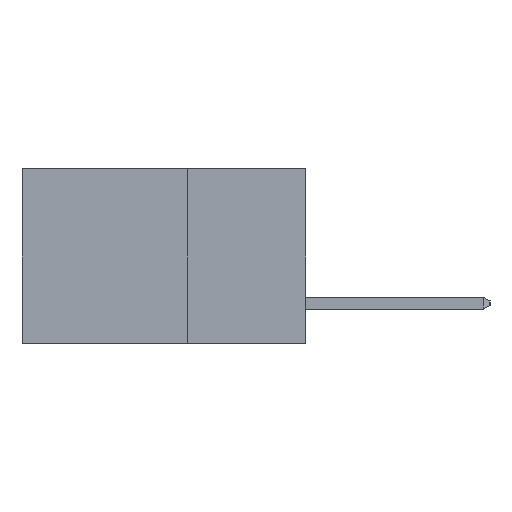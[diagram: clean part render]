
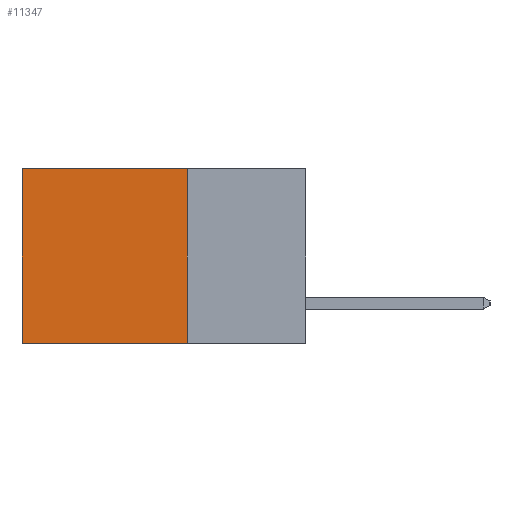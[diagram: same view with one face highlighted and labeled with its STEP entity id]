
A CAD part, left-side view. The second image highlights one B-rep face of the part: STEP entity #11347.
In plain terms, the highlighted planar face has unit normal (-1, 0, 0).
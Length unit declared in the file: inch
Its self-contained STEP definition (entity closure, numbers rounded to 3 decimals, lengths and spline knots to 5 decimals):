
#535 = EDGE_LOOP ( 'NONE', ( #16346, #4871, #7516, #13680 ) ) ;
#562 = CARTESIAN_POINT ( 'NONE',  ( 0.2615, 0.25, 0. ) ) ;
#1863 = EDGE_CURVE ( 'NONE', #21074, #2598, #10101, .T. ) ;
#2318 = CARTESIAN_POINT ( 'NONE',  ( 0.2615, 0.6, 0. ) ) ;
#2598 = VERTEX_POINT ( 'NONE', #2318 ) ;
#2618 = FACE_OUTER_BOUND ( 'NONE', #535, .T. ) ;
#3104 = CARTESIAN_POINT ( 'NONE',  ( 0.2615, 0.25, -0.37 ) ) ;
#3244 = VECTOR ( 'NONE', #5873, 39.37008 ) ;
#3981 = EDGE_CURVE ( 'NONE', #2598, #5927, #22085, .T. ) ;
#4871 = ORIENTED_EDGE ( 'NONE', *, *, #16105, .F. ) ;
#4941 = DIRECTION ( 'NONE',  ( 0., 0., -1. ) ) ;
#5873 = DIRECTION ( 'NONE',  ( 0., 0., -1. ) ) ;
#5927 = VERTEX_POINT ( 'NONE', #10824 ) ;
#7516 = ORIENTED_EDGE ( 'NONE', *, *, #17781, .F. ) ;
#10101 = LINE ( 'NONE', #17172, #18935 ) ;
#10824 = CARTESIAN_POINT ( 'NONE',  ( 0.2615, 0.6, -0.37 ) ) ;
#11130 = VECTOR ( 'NONE', #15804, 39.37008 ) ;
#11347 = ADVANCED_FACE ( 'NONE', ( #2618 ), #18997, .F. ) ;
#12167 = LINE ( 'NONE', #16474, #3244 ) ;
#13680 = ORIENTED_EDGE ( 'NONE', *, *, #1863, .T. ) ;
#14666 = VERTEX_POINT ( 'NONE', #17314 ) ;
#15548 = DIRECTION ( 'NONE',  ( 1., 0., 0. ) ) ;
#15804 = DIRECTION ( 'NONE',  ( 0., 1., 0. ) ) ;
#15855 = LINE ( 'NONE', #19243, #11130 ) ;
#16105 = EDGE_CURVE ( 'NONE', #14666, #5927, #15855, .T. ) ;
#16346 = ORIENTED_EDGE ( 'NONE', *, *, #3981, .T. ) ;
#16474 = CARTESIAN_POINT ( 'NONE',  ( 0.2615, 0.25, -0.37 ) ) ;
#17172 = CARTESIAN_POINT ( 'NONE',  ( 0.2615, 0.25, 0. ) ) ;
#17279 = DIRECTION ( 'NONE',  ( 0., 1., 0. ) ) ;
#17314 = CARTESIAN_POINT ( 'NONE',  ( 0.2615, 0.25, -0.37 ) ) ;
#17781 = EDGE_CURVE ( 'NONE', #21074, #14666, #12167, .T. ) ;
#18935 = VECTOR ( 'NONE', #17279, 39.37008 ) ;
#18997 = PLANE ( 'NONE',  #20192 ) ;
#19208 = VECTOR ( 'NONE', #22179, 39.37008 ) ;
#19243 = CARTESIAN_POINT ( 'NONE',  ( 0.2615, 0.25, -0.37 ) ) ;
#20192 = AXIS2_PLACEMENT_3D ( 'NONE', #3104, #15548, #4941 ) ;
#21074 = VERTEX_POINT ( 'NONE', #562 ) ;
#22085 = LINE ( 'NONE', #22615, #19208 ) ;
#22179 = DIRECTION ( 'NONE',  ( 0., 0., -1. ) ) ;
#22615 = CARTESIAN_POINT ( 'NONE',  ( 0.2615, 0.6, -0.37 ) ) ;
